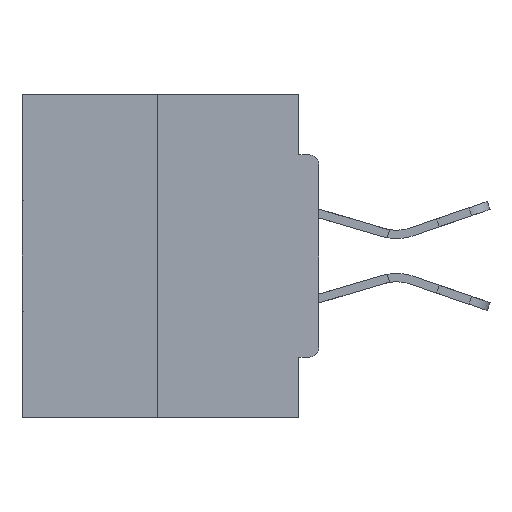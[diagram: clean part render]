
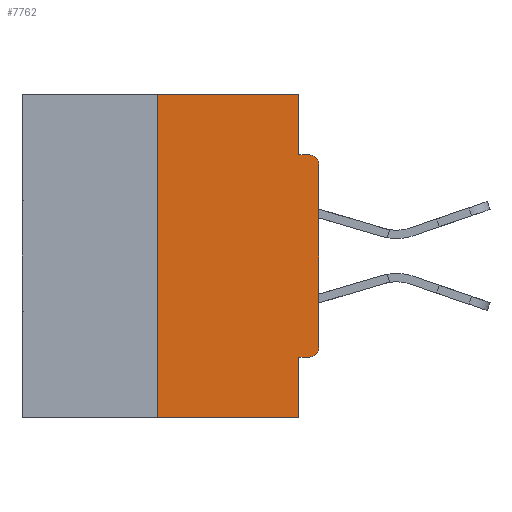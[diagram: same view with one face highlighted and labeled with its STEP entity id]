
A CAD part, left-side view. The second image highlights one B-rep face of the part: STEP entity #7762.
In plain terms, the highlighted planar face has unit normal (-1, 0, 0).
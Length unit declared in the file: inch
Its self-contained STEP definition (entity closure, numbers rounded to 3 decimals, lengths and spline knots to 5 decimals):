
#861 = CARTESIAN_POINT ( 'NONE',  ( 0., 0.46, 0. ) ) ;
#1239 = EDGE_CURVE ( 'NONE', #21567, #38872, #19009, .T. ) ;
#1440 = DIRECTION ( 'NONE',  ( 0., 0., 1. ) ) ;
#1614 = DIRECTION ( 'NONE',  ( 0., -1., 0. ) ) ;
#1864 = CARTESIAN_POINT ( 'NONE',  ( 0., 0.25, -0.5 ) ) ;
#2764 = CIRCLE ( 'NONE', #13925, 0.015 ) ;
#3619 = VECTOR ( 'NONE', #24350, 39.37008 ) ;
#5736 = EDGE_CURVE ( 'NONE', #38872, #10688, #19747, .T. ) ;
#5950 = CARTESIAN_POINT ( 'NONE',  ( 0., 0.46, 0. ) ) ;
#6094 = CARTESIAN_POINT ( 'NONE',  ( 0., 0.015, -0.1085 ) ) ;
#6229 = DIRECTION ( 'NONE',  ( 0., -1., 0. ) ) ;
#6507 = ORIENTED_EDGE ( 'NONE', *, *, #37308, .F. ) ;
#7219 = LINE ( 'NONE', #37575, #21227 ) ;
#7319 = DIRECTION ( 'NONE',  ( 0., 0., -1. ) ) ;
#7450 = CARTESIAN_POINT ( 'NONE',  ( 0., 0., -0.4065 ) ) ;
#7588 = CARTESIAN_POINT ( 'NONE',  ( 0., 0.25, 0. ) ) ;
#7647 = ORIENTED_EDGE ( 'NONE', *, *, #8915, .T. ) ;
#7762 = ADVANCED_FACE ( 'NONE', ( #8631 ), #29257, .F. ) ;
#8631 = FACE_OUTER_BOUND ( 'NONE', #34052, .T. ) ;
#8915 = EDGE_CURVE ( 'NONE', #21567, #12066, #15570, .T. ) ;
#9036 = EDGE_CURVE ( 'NONE', #38278, #12066, #13536, .T. ) ;
#9294 = DIRECTION ( 'NONE',  ( 0., 0., -1. ) ) ;
#10226 = CARTESIAN_POINT ( 'NONE',  ( 0., 0., -0.1085 ) ) ;
#10467 = CARTESIAN_POINT ( 'NONE',  ( 0., 0.031, -0.5 ) ) ;
#10688 = VERTEX_POINT ( 'NONE', #27525 ) ;
#11759 = DIRECTION ( 'NONE',  ( 0., 0., -1. ) ) ;
#12066 = VERTEX_POINT ( 'NONE', #10467 ) ;
#12574 = LINE ( 'NONE', #30706, #38132 ) ;
#13086 = CARTESIAN_POINT ( 'NONE',  ( 0., 0.015, -0.0935 ) ) ;
#13536 = LINE ( 'NONE', #27661, #41087 ) ;
#13925 = AXIS2_PLACEMENT_3D ( 'NONE', #30470, #23769, #14502 ) ;
#14502 = DIRECTION ( 'NONE',  ( 0., 0., -1. ) ) ;
#14642 = EDGE_CURVE ( 'NONE', #37687, #32021, #22091, .T. ) ;
#15301 = DIRECTION ( 'NONE',  ( 0., 0., -1. ) ) ;
#15570 = LINE ( 'NONE', #34665, #17543 ) ;
#15815 = AXIS2_PLACEMENT_3D ( 'NONE', #6094, #28435, #9294 ) ;
#17543 = VECTOR ( 'NONE', #31294, 39.37008 ) ;
#17791 = ORIENTED_EDGE ( 'NONE', *, *, #9036, .F. ) ;
#18379 = CARTESIAN_POINT ( 'NONE',  ( 0., 0., -0.3915 ) ) ;
#18428 = CARTESIAN_POINT ( 'NONE',  ( 0., 0.25, 0. ) ) ;
#19009 = LINE ( 'NONE', #7588, #22520 ) ;
#19747 = LINE ( 'NONE', #5950, #26253 ) ;
#20624 = LINE ( 'NONE', #36665, #3619 ) ;
#21227 = VECTOR ( 'NONE', #15301, 39.37008 ) ;
#21567 = VERTEX_POINT ( 'NONE', #1864 ) ;
#22091 = CIRCLE ( 'NONE', #15815, 0.015 ) ;
#22520 = VECTOR ( 'NONE', #1440, 39.37008 ) ;
#22646 = AXIS2_PLACEMENT_3D ( 'NONE', #861, #38964, #7319 ) ;
#23769 = DIRECTION ( 'NONE',  ( -1., 0., 0. ) ) ;
#24190 = ORIENTED_EDGE ( 'NONE', *, *, #1239, .F. ) ;
#24350 = DIRECTION ( 'NONE',  ( 0., 0., 1. ) ) ;
#26033 = EDGE_CURVE ( 'NONE', #29359, #37687, #20624, .T. ) ;
#26253 = VECTOR ( 'NONE', #6229, 39.37008 ) ;
#27525 = CARTESIAN_POINT ( 'NONE',  ( 0., 0.031, 0. ) ) ;
#27661 = CARTESIAN_POINT ( 'NONE',  ( 0., 0.031, -0.5 ) ) ;
#27730 = VERTEX_POINT ( 'NONE', #35463 ) ;
#27755 = ORIENTED_EDGE ( 'NONE', *, *, #26033, .T. ) ;
#28435 = DIRECTION ( 'NONE',  ( -1., 0., 0. ) ) ;
#28472 = CARTESIAN_POINT ( 'NONE',  ( 0., 0.031, -0.4065 ) ) ;
#29257 = PLANE ( 'NONE',  #22646 ) ;
#29359 = VERTEX_POINT ( 'NONE', #18379 ) ;
#30470 = CARTESIAN_POINT ( 'NONE',  ( 0., 0.015, -0.3915 ) ) ;
#30706 = CARTESIAN_POINT ( 'NONE',  ( 0., 0., -0.0935 ) ) ;
#31294 = DIRECTION ( 'NONE',  ( 0., -1., 0. ) ) ;
#32021 = VERTEX_POINT ( 'NONE', #13086 ) ;
#32119 = VECTOR ( 'NONE', #39795, 39.37008 ) ;
#33362 = ORIENTED_EDGE ( 'NONE', *, *, #5736, .F. ) ;
#34052 = EDGE_LOOP ( 'NONE', ( #33362, #24190, #7647, #17791, #6507, #39372, #27755, #34283, #40319, #36672 ) ) ;
#34283 = ORIENTED_EDGE ( 'NONE', *, *, #14642, .T. ) ;
#34665 = CARTESIAN_POINT ( 'NONE',  ( 0., 0.46, -0.5 ) ) ;
#35463 = CARTESIAN_POINT ( 'NONE',  ( 0., 0.015, -0.4065 ) ) ;
#36665 = CARTESIAN_POINT ( 'NONE',  ( 0., 0., 0. ) ) ;
#36672 = ORIENTED_EDGE ( 'NONE', *, *, #41383, .F. ) ;
#37308 = EDGE_CURVE ( 'NONE', #27730, #38278, #40643, .T. ) ;
#37575 = CARTESIAN_POINT ( 'NONE',  ( 0., 0.031, 0. ) ) ;
#37687 = VERTEX_POINT ( 'NONE', #10226 ) ;
#38132 = VECTOR ( 'NONE', #1614, 39.37008 ) ;
#38278 = VERTEX_POINT ( 'NONE', #28472 ) ;
#38872 = VERTEX_POINT ( 'NONE', #18428 ) ;
#38964 = DIRECTION ( 'NONE',  ( 1., 0., 0. ) ) ;
#39372 = ORIENTED_EDGE ( 'NONE', *, *, #41009, .T. ) ;
#39716 = VERTEX_POINT ( 'NONE', #40255 ) ;
#39765 = EDGE_CURVE ( 'NONE', #39716, #32021, #12574, .T. ) ;
#39795 = DIRECTION ( 'NONE',  ( 0., 1., 0. ) ) ;
#40255 = CARTESIAN_POINT ( 'NONE',  ( 0., 0.031, -0.0935 ) ) ;
#40319 = ORIENTED_EDGE ( 'NONE', *, *, #39765, .F. ) ;
#40643 = LINE ( 'NONE', #7450, #32119 ) ;
#41009 = EDGE_CURVE ( 'NONE', #27730, #29359, #2764, .T. ) ;
#41087 = VECTOR ( 'NONE', #11759, 39.37008 ) ;
#41383 = EDGE_CURVE ( 'NONE', #10688, #39716, #7219, .T. ) ;
